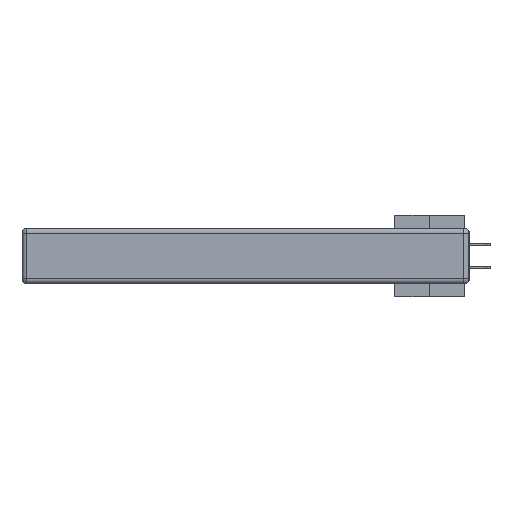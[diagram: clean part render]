
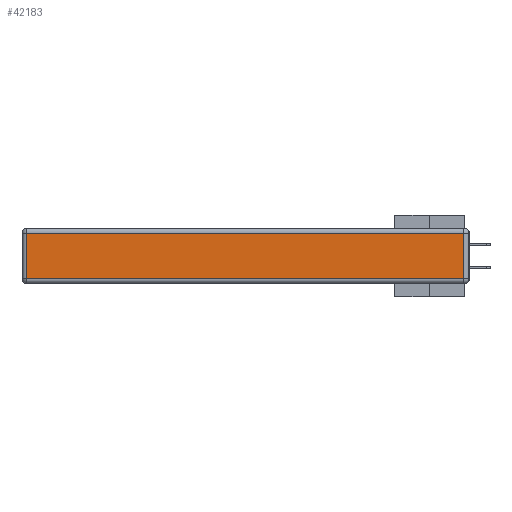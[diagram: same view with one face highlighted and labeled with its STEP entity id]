
A CAD part, left-side view. The second image highlights one B-rep face of the part: STEP entity #42183.
In plain terms, the highlighted planar face has unit normal (-1, 0, 0).
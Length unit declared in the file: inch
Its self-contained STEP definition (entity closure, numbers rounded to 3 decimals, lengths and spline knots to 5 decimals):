
#234 = ORIENTED_EDGE ( 'NONE', *, *, #36156, .T. ) ;
#2570 = VERTEX_POINT ( 'NONE', #14129 ) ;
#7642 = ORIENTED_EDGE ( 'NONE', *, *, #19770, .T. ) ;
#8188 = CARTESIAN_POINT ( 'NONE',  ( 0., 2.72, -0.03 ) ) ;
#8632 = DIRECTION ( 'NONE',  ( 0., 1., 0. ) ) ;
#8799 = EDGE_CURVE ( 'NONE', #2570, #36927, #41219, .T. ) ;
#8948 = CARTESIAN_POINT ( 'NONE',  ( 0., 2.75, -0.03 ) ) ;
#10492 = DIRECTION ( 'NONE',  ( -1., 0., 0. ) ) ;
#12782 = VECTOR ( 'NONE', #8632, 39.37008 ) ;
#13706 = AXIS2_PLACEMENT_3D ( 'NONE', #32966, #10492, #25150 ) ;
#14129 = CARTESIAN_POINT ( 'NONE',  ( 0., 2.72, -0.313 ) ) ;
#14819 = CARTESIAN_POINT ( 'NONE',  ( 0., 0., -0.313 ) ) ;
#17274 = VERTEX_POINT ( 'NONE', #36109 ) ;
#19108 = DIRECTION ( 'NONE',  ( 0., -1., 0. ) ) ;
#19389 = LINE ( 'NONE', #34761, #46221 ) ;
#19770 = EDGE_CURVE ( 'NONE', #25989, #2570, #19389, .T. ) ;
#21715 = DIRECTION ( 'NONE',  ( 0., 0., 1. ) ) ;
#22334 = CARTESIAN_POINT ( 'NONE',  ( 0., 0.03, -0.343 ) ) ;
#24206 = CARTESIAN_POINT ( 'NONE',  ( 0., 0.03, -0.313 ) ) ;
#24682 = EDGE_CURVE ( 'NONE', #36927, #17274, #41123, .T. ) ;
#25150 = DIRECTION ( 'NONE',  ( 0., 0., 1. ) ) ;
#25983 = ORIENTED_EDGE ( 'NONE', *, *, #24682, .T. ) ;
#25989 = VERTEX_POINT ( 'NONE', #8188 ) ;
#31497 = VECTOR ( 'NONE', #19108, 39.37008 ) ;
#32892 = ORIENTED_EDGE ( 'NONE', *, *, #8799, .T. ) ;
#32966 = CARTESIAN_POINT ( 'NONE',  ( 0., 0., -0.343 ) ) ;
#34761 = CARTESIAN_POINT ( 'NONE',  ( 0., 2.72, -0.343 ) ) ;
#35924 = DIRECTION ( 'NONE',  ( 0., 0., -1. ) ) ;
#36109 = CARTESIAN_POINT ( 'NONE',  ( 0., 0.03, -0.03 ) ) ;
#36156 = EDGE_CURVE ( 'NONE', #17274, #25989, #47024, .T. ) ;
#36927 = VERTEX_POINT ( 'NONE', #24206 ) ;
#37358 = EDGE_LOOP ( 'NONE', ( #32892, #25983, #234, #7642 ) ) ;
#38909 = FACE_OUTER_BOUND ( 'NONE', #37358, .T. ) ;
#41123 = LINE ( 'NONE', #22334, #42297 ) ;
#41219 = LINE ( 'NONE', #14819, #31497 ) ;
#42183 = ADVANCED_FACE ( 'NONE', ( #38909 ), #47029, .T. ) ;
#42297 = VECTOR ( 'NONE', #21715, 39.37008 ) ;
#46221 = VECTOR ( 'NONE', #35924, 39.37008 ) ;
#47024 = LINE ( 'NONE', #8948, #12782 ) ;
#47029 = PLANE ( 'NONE',  #13706 ) ;
